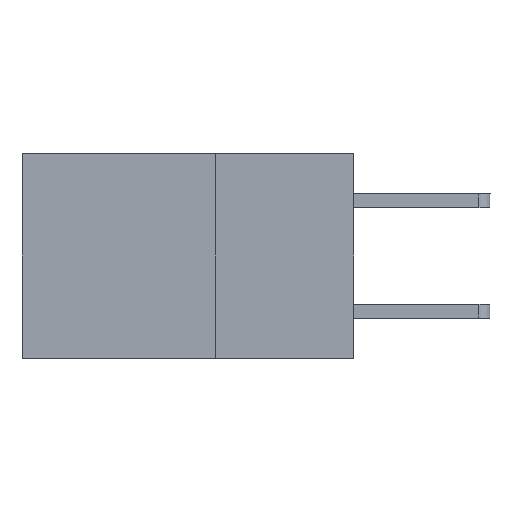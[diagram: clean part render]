
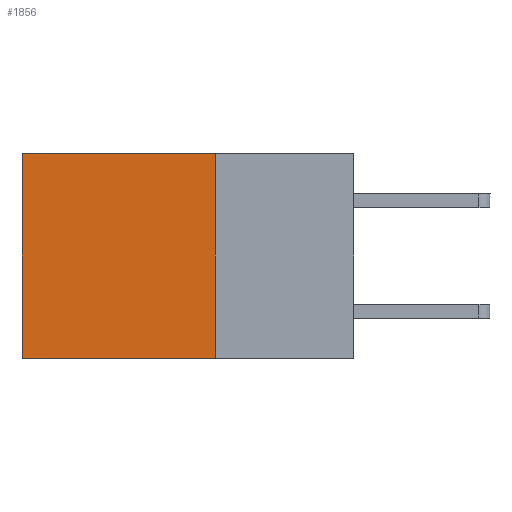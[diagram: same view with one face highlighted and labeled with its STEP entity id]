
A CAD part, left-side view. The second image highlights one B-rep face of the part: STEP entity #1856.
In plain terms, the highlighted planar face has unit normal (-1, 0, 0).
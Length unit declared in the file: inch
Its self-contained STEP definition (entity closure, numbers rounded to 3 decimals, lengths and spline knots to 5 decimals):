
#272 = VECTOR ( 'NONE', #8572, 39.37008 ) ;
#276 = CARTESIAN_POINT ( 'NONE',  ( 0.2875, 0.25, 0. ) ) ;
#301 = VERTEX_POINT ( 'NONE', #276 ) ;
#671 = EDGE_LOOP ( 'NONE', ( #3298, #3405, #3432, #3492 ) ) ;
#1151 = PLANE ( 'NONE',  #1965 ) ;
#1172 = DIRECTION ( 'NONE',  ( 0., 0., -1. ) ) ;
#1311 = VECTOR ( 'NONE', #7096, 39.37008 ) ;
#1359 = VERTEX_POINT ( 'NONE', #8625 ) ;
#1791 = LINE ( 'NONE', #4435, #8523 ) ;
#1856 = ADVANCED_FACE ( 'NONE', ( #4618 ), #1151, .F. ) ;
#1965 = AXIS2_PLACEMENT_3D ( 'NONE', #6208, #6693, #1172 ) ;
#2272 = EDGE_CURVE ( 'NONE', #8688, #6259, #7028, .T. ) ;
#2796 = LINE ( 'NONE', #6737, #272 ) ;
#3154 = CARTESIAN_POINT ( 'NONE',  ( 0.2875, 0.6, -0.37 ) ) ;
#3298 = ORIENTED_EDGE ( 'NONE', *, *, #4418, .T. ) ;
#3405 = ORIENTED_EDGE ( 'NONE', *, *, #2272, .F. ) ;
#3432 = ORIENTED_EDGE ( 'NONE', *, *, #6354, .F. ) ;
#3439 = EDGE_CURVE ( 'NONE', #301, #1359, #1791, .T. ) ;
#3489 = CARTESIAN_POINT ( 'NONE',  ( 0.2875, 0.25, -0.37 ) ) ;
#3492 = ORIENTED_EDGE ( 'NONE', *, *, #3439, .T. ) ;
#3508 = DIRECTION ( 'NONE',  ( 0., 1., 0. ) ) ;
#4418 = EDGE_CURVE ( 'NONE', #1359, #6259, #2796, .T. ) ;
#4435 = CARTESIAN_POINT ( 'NONE',  ( 0.2875, 0.25, 0. ) ) ;
#4618 = FACE_OUTER_BOUND ( 'NONE', #671, .T. ) ;
#4771 = DIRECTION ( 'NONE',  ( 0., 1., 0. ) ) ;
#5278 = CARTESIAN_POINT ( 'NONE',  ( 0.2875, 0.25, 0. ) ) ;
#6208 = CARTESIAN_POINT ( 'NONE',  ( 0.2875, 0.25, 0. ) ) ;
#6259 = VERTEX_POINT ( 'NONE', #3154 ) ;
#6354 = EDGE_CURVE ( 'NONE', #301, #8688, #6765, .T. ) ;
#6693 = DIRECTION ( 'NONE',  ( 1., 0., 0. ) ) ;
#6737 = CARTESIAN_POINT ( 'NONE',  ( 0.2875, 0.6, 0. ) ) ;
#6765 = LINE ( 'NONE', #5278, #1311 ) ;
#7028 = LINE ( 'NONE', #3489, #7211 ) ;
#7096 = DIRECTION ( 'NONE',  ( 0., 0., -1. ) ) ;
#7211 = VECTOR ( 'NONE', #3508, 39.37008 ) ;
#8367 = CARTESIAN_POINT ( 'NONE',  ( 0.2875, 0.25, -0.37 ) ) ;
#8523 = VECTOR ( 'NONE', #4771, 39.37008 ) ;
#8572 = DIRECTION ( 'NONE',  ( 0., 0., -1. ) ) ;
#8625 = CARTESIAN_POINT ( 'NONE',  ( 0.2875, 0.6, 0. ) ) ;
#8688 = VERTEX_POINT ( 'NONE', #8367 ) ;
